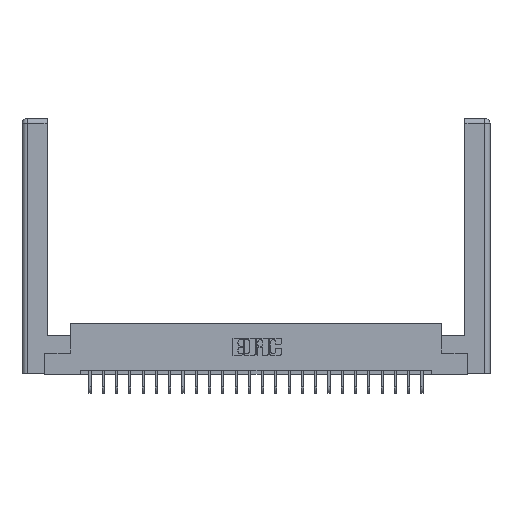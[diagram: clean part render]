
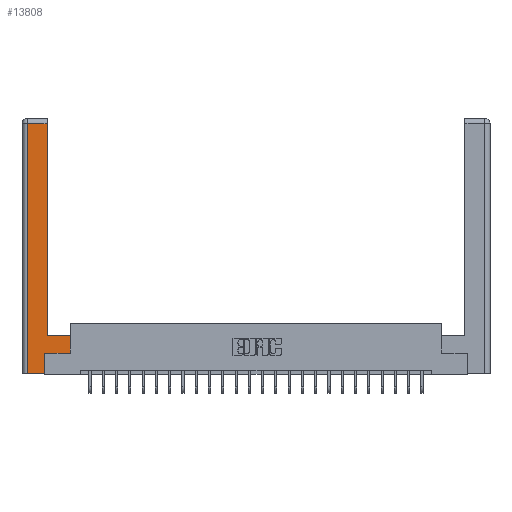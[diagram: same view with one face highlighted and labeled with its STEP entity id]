
A CAD part, top view. The second image highlights one B-rep face of the part: STEP entity #13808.
In plain terms, the highlighted planar face has unit normal (0, 0, 1).
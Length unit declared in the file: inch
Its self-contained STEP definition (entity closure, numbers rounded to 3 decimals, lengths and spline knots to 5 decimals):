
#8 = VECTOR ( 'NONE', #2641, 39.37008 ) ;
#9 = EDGE_CURVE ( 'NONE', #9851, #23226, #4973, .T. ) ;
#134 = CARTESIAN_POINT ( 'NONE',  ( 0.295, 2.94, 0. ) ) ;
#209 = LINE ( 'NONE', #12007, #22760 ) ;
#382 = ORIENTED_EDGE ( 'NONE', *, *, #23629, .T. ) ;
#641 = VERTEX_POINT ( 'NONE', #22276 ) ;
#1551 = ORIENTED_EDGE ( 'NONE', *, *, #11824, .T. ) ;
#2092 = VERTEX_POINT ( 'NONE', #17294 ) ;
#2641 = DIRECTION ( 'NONE',  ( 0., 1., 0. ) ) ;
#2779 = FACE_OUTER_BOUND ( 'NONE', #4536, .T. ) ;
#3223 = CARTESIAN_POINT ( 'NONE',  ( 0.265, 0., 0. ) ) ;
#4232 = LINE ( 'NONE', #13181, #24152 ) ;
#4258 = AXIS2_PLACEMENT_3D ( 'NONE', #11378, #21423, #5262 ) ;
#4304 = CARTESIAN_POINT ( 'NONE',  ( 0.265, 0., 0. ) ) ;
#4536 = EDGE_LOOP ( 'NONE', ( #6119, #23524, #16840, #14830, #10989, #14116, #382, #1551 ) ) ;
#4648 = EDGE_CURVE ( 'NONE', #641, #9851, #209, .T. ) ;
#4931 = EDGE_CURVE ( 'NONE', #24910, #2092, #6360, .T. ) ;
#4973 = LINE ( 'NONE', #4304, #6256 ) ;
#4977 = DIRECTION ( 'NONE',  ( 1., 0., 0. ) ) ;
#5047 = DIRECTION ( 'NONE',  ( 0., 1., 0. ) ) ;
#5262 = DIRECTION ( 'NONE',  ( -1., 0., 0. ) ) ;
#5492 = EDGE_CURVE ( 'NONE', #13653, #21543, #6506, .T. ) ;
#5514 = LINE ( 'NONE', #18913, #8 ) ;
#5806 = VECTOR ( 'NONE', #13847, 39.37008 ) ;
#6119 = ORIENTED_EDGE ( 'NONE', *, *, #5492, .T. ) ;
#6133 = CARTESIAN_POINT ( 'NONE',  ( 0.565, 0.45, 0. ) ) ;
#6256 = VECTOR ( 'NONE', #16794, 39.37008 ) ;
#6360 = LINE ( 'NONE', #23659, #24976 ) ;
#6499 = EDGE_CURVE ( 'NONE', #21543, #641, #4232, .T. ) ;
#6506 = LINE ( 'NONE', #21573, #7471 ) ;
#7471 = VECTOR ( 'NONE', #5047, 39.37008 ) ;
#7793 = VECTOR ( 'NONE', #22053, 39.37008 ) ;
#9851 = VERTEX_POINT ( 'NONE', #11485 ) ;
#9973 = CARTESIAN_POINT ( 'NONE',  ( 0.295, 0.45, 0. ) ) ;
#10989 = ORIENTED_EDGE ( 'NONE', *, *, #15985, .T. ) ;
#11291 = VERTEX_POINT ( 'NONE', #6133 ) ;
#11378 = CARTESIAN_POINT ( 'NONE',  ( 0., 0., 0. ) ) ;
#11384 = DIRECTION ( 'NONE',  ( -1., 0., 0. ) ) ;
#11407 = CARTESIAN_POINT ( 'NONE',  ( 0.265, 0.245, 0. ) ) ;
#11485 = CARTESIAN_POINT ( 'NONE',  ( 0.0615, 0., 0. ) ) ;
#11824 = EDGE_CURVE ( 'NONE', #11291, #13653, #22517, .T. ) ;
#12007 = CARTESIAN_POINT ( 'NONE',  ( 0.0615, 0., 0. ) ) ;
#13181 = CARTESIAN_POINT ( 'NONE',  ( 0.0615, 2.94, 0. ) ) ;
#13653 = VERTEX_POINT ( 'NONE', #9973 ) ;
#13808 = ADVANCED_FACE ( 'NONE', ( #2779 ), #19005, .F. ) ;
#13847 = DIRECTION ( 'NONE',  ( -1., 0., 0. ) ) ;
#14116 = ORIENTED_EDGE ( 'NONE', *, *, #4931, .T. ) ;
#14830 = ORIENTED_EDGE ( 'NONE', *, *, #9, .T. ) ;
#15820 = CARTESIAN_POINT ( 'NONE',  ( 0.295, 0.45, 0. ) ) ;
#15985 = EDGE_CURVE ( 'NONE', #23226, #24910, #16817, .T. ) ;
#16794 = DIRECTION ( 'NONE',  ( 1., 0., 0. ) ) ;
#16817 = LINE ( 'NONE', #11407, #7793 ) ;
#16840 = ORIENTED_EDGE ( 'NONE', *, *, #4648, .T. ) ;
#17294 = CARTESIAN_POINT ( 'NONE',  ( 0.565, 0.245, 0. ) ) ;
#18913 = CARTESIAN_POINT ( 'NONE',  ( 0.565, 0.45, 0. ) ) ;
#19005 = PLANE ( 'NONE',  #4258 ) ;
#21085 = CARTESIAN_POINT ( 'NONE',  ( 0.265, 0.245, 0. ) ) ;
#21423 = DIRECTION ( 'NONE',  ( 0., 0., -1. ) ) ;
#21543 = VERTEX_POINT ( 'NONE', #134 ) ;
#21573 = CARTESIAN_POINT ( 'NONE',  ( 0.295, 3., 0. ) ) ;
#22053 = DIRECTION ( 'NONE',  ( 0., 1., 0. ) ) ;
#22276 = CARTESIAN_POINT ( 'NONE',  ( 0.0615, 2.94, 0. ) ) ;
#22517 = LINE ( 'NONE', #15820, #5806 ) ;
#22760 = VECTOR ( 'NONE', #26395, 39.37008 ) ;
#23226 = VERTEX_POINT ( 'NONE', #3223 ) ;
#23524 = ORIENTED_EDGE ( 'NONE', *, *, #6499, .T. ) ;
#23629 = EDGE_CURVE ( 'NONE', #2092, #11291, #5514, .T. ) ;
#23659 = CARTESIAN_POINT ( 'NONE',  ( 0.565, 0.245, 0. ) ) ;
#24152 = VECTOR ( 'NONE', #11384, 39.37008 ) ;
#24910 = VERTEX_POINT ( 'NONE', #21085 ) ;
#24976 = VECTOR ( 'NONE', #4977, 39.37008 ) ;
#26395 = DIRECTION ( 'NONE',  ( 0., -1., 0. ) ) ;
